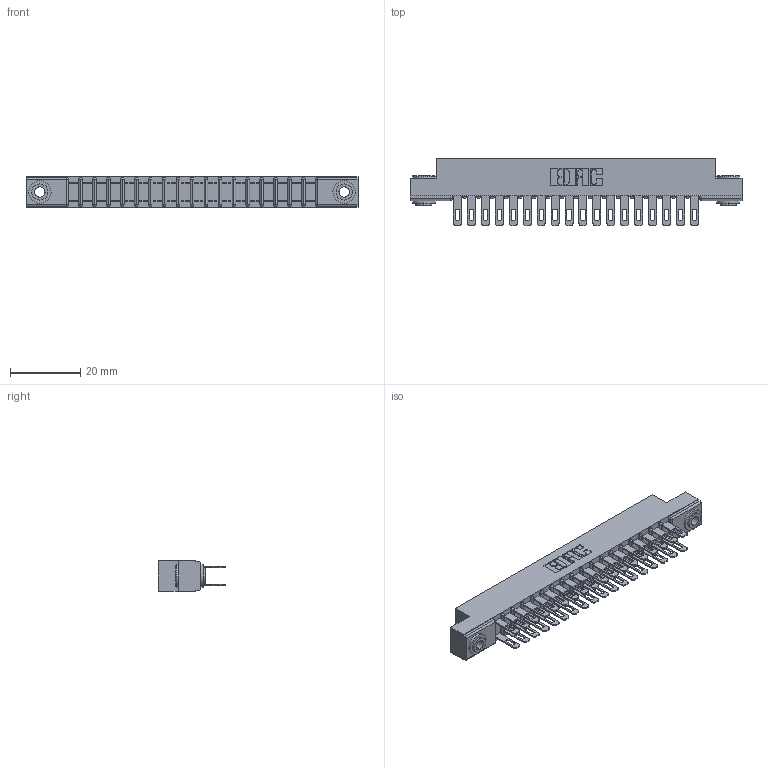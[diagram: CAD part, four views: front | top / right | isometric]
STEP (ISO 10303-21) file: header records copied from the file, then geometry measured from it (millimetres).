
FILE_DESCRIPTION (( 'STEP AP203' ), '1' );
FILE_NAME ('307-036-500-203.STEP', '2019-09-06T03:06:50', ( '' ), ( '' ), 'SwSTEP 2.0', 'SolidWorks 2016', '' );
FILE_SCHEMA (( 'CONFIG_CONTROL_DESIGN' ));
Length unit declared in the file: inch
Products named in the file (4): 345-250-002_345-250-002-102; 307 Part_.156 Dia Mounting Holes; 307-290-001_500; 307-036-500-203
Assembly tree (39 placements, depth 2):
  307-036-500-203
    307 Part_.156 Dia Mounting Holes
    307-290-001_500  x36
    345-250-002_345-250-002-102  x2
Bounding box: 94.34 x 19.18 x 8.71 mm (x, y, z)
Volume: 6275.5 mm3; surface area: 11694.9 mm2
Topology: 39 solids, 39 shells, 1845 faces, 5115 edges, 3306 vertices
Faces by surface type: plane 1174, cylinder 625, sphere 38, cone 8
Entity records: 20005 total; most frequent: CARTESIAN_POINT 3259, DIRECTION 3219, ORIENTED_EDGE 3218, EDGE_CURVE 1609, VECTOR 1215, LINE 1215, VERTEX_POINT 1042, AXIS2_PLACEMENT_3D 1002
